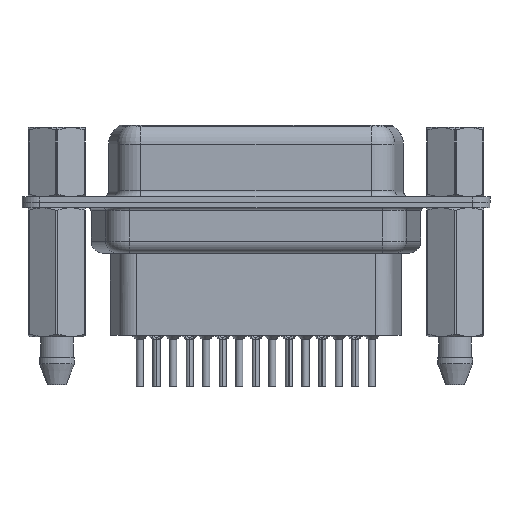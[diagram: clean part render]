
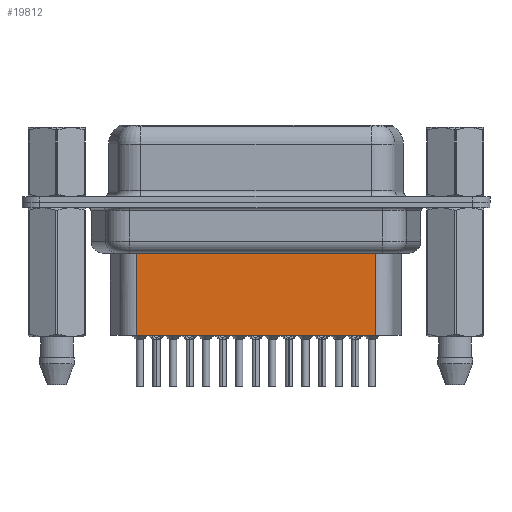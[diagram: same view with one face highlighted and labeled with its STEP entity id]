
A CAD part, front view. The second image highlights one B-rep face of the part: STEP entity #19812.
In plain terms, the highlighted planar face has unit normal (0, -1, 0).
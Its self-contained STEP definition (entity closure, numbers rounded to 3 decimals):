
#4320 = CARTESIAN_POINT ( 'NONE',  ( 6.681, -3.5, -11.15 ) ) ;
#5275 = DIRECTION ( 'NONE',  ( 0., 0., -1. ) ) ;
#5485 = DIRECTION ( 'NONE',  ( 0., 0., -1. ) ) ;
#5539 = DIRECTION ( 'NONE',  ( -1., 0., 0. ) ) ;
#6074 = FACE_OUTER_BOUND ( 'NONE', #6376, .T. ) ;
#6376 = EDGE_LOOP ( 'NONE', ( #7860, #24601, #8570, #21725 ) ) ;
#6927 = LINE ( 'NONE', #23196, #24209 ) ;
#7219 = EDGE_CURVE ( 'NONE', #13150, #12985, #29006, .T. ) ;
#7860 = ORIENTED_EDGE ( 'NONE', *, *, #26360, .F. ) ;
#7936 = CARTESIAN_POINT ( 'NONE',  ( 6.681, -3.5, -4.097 ) ) ;
#8122 = LINE ( 'NONE', #16036, #13133 ) ;
#8137 = VECTOR ( 'NONE', #8304, 1000. ) ;
#8304 = DIRECTION ( 'NONE',  ( -1., 0., 0. ) ) ;
#8426 = CARTESIAN_POINT ( 'NONE',  ( 26.619, -3.5, -4.097 ) ) ;
#8570 = ORIENTED_EDGE ( 'NONE', *, *, #28264, .T. ) ;
#10807 = CARTESIAN_POINT ( 'NONE',  ( 6.681, -3.5, -11.15 ) ) ;
#11439 = CARTESIAN_POINT ( 'NONE',  ( 6.434, -3.5, -4.097 ) ) ;
#12985 = VERTEX_POINT ( 'NONE', #7936 ) ;
#13133 = VECTOR ( 'NONE', #5485, 1000. ) ;
#13150 = VERTEX_POINT ( 'NONE', #8426 ) ;
#16036 = CARTESIAN_POINT ( 'NONE',  ( 26.619, -3.5, -3.1 ) ) ;
#16141 = DIRECTION ( 'NONE',  ( 1., 0., 0. ) ) ;
#19812 = ADVANCED_FACE ( 'NONE', ( #6074 ), #23988, .T. ) ;
#21383 = CARTESIAN_POINT ( 'NONE',  ( 6.681, -3.5, -3.1 ) ) ;
#21725 = ORIENTED_EDGE ( 'NONE', *, *, #24690, .F. ) ;
#23196 = CARTESIAN_POINT ( 'NONE',  ( 6.681, -3.5, -3.1 ) ) ;
#23665 = DIRECTION ( 'NONE',  ( 0., -1., 0. ) ) ;
#23988 = PLANE ( 'NONE',  #26568 ) ;
#24202 = VERTEX_POINT ( 'NONE', #4320 ) ;
#24209 = VECTOR ( 'NONE', #5275, 1000. ) ;
#24601 = ORIENTED_EDGE ( 'NONE', *, *, #7219, .T. ) ;
#24690 = EDGE_CURVE ( 'NONE', #30221, #24202, #26073, .T. ) ;
#26073 = LINE ( 'NONE', #10807, #31943 ) ;
#26360 = EDGE_CURVE ( 'NONE', #13150, #30221, #8122, .T. ) ;
#26568 = AXIS2_PLACEMENT_3D ( 'NONE', #21383, #23665, #16141 ) ;
#28264 = EDGE_CURVE ( 'NONE', #12985, #24202, #6927, .T. ) ;
#29006 = LINE ( 'NONE', #11439, #8137 ) ;
#30221 = VERTEX_POINT ( 'NONE', #30720 ) ;
#30720 = CARTESIAN_POINT ( 'NONE',  ( 26.619, -3.5, -11.15 ) ) ;
#31943 = VECTOR ( 'NONE', #5539, 1000. ) ;
